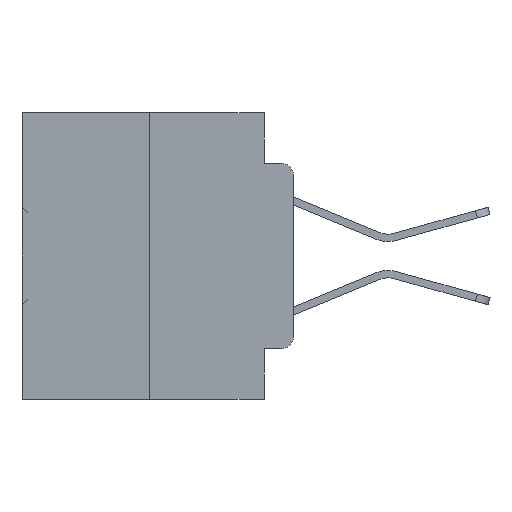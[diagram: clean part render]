
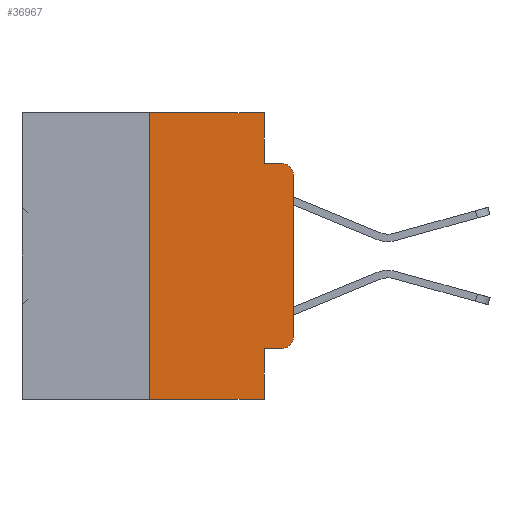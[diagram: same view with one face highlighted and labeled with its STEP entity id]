
A CAD part, left-side view. The second image highlights one B-rep face of the part: STEP entity #36967.
In plain terms, the highlighted planar face has unit normal (-1, 0, 0).
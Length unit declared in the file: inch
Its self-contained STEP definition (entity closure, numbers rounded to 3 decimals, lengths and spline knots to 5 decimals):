
#874 = AXIS2_PLACEMENT_3D ( 'NONE', #28032, #21718, #24745 ) ;
#1392 = VERTEX_POINT ( 'NONE', #15506 ) ;
#1552 = DIRECTION ( 'NONE',  ( 0., -1., 0. ) ) ;
#2329 = VERTEX_POINT ( 'NONE', #30217 ) ;
#2454 = CARTESIAN_POINT ( 'NONE',  ( 0., 0., 0. ) ) ;
#2911 = VECTOR ( 'NONE', #18882, 39.37008 ) ;
#3037 = ORIENTED_EDGE ( 'NONE', *, *, #19415, .F. ) ;
#3250 = CARTESIAN_POINT ( 'NONE',  ( 0., 0.473, -0.5 ) ) ;
#3820 = LINE ( 'NONE', #2454, #37466 ) ;
#4204 = PLANE ( 'NONE',  #874 ) ;
#4285 = CARTESIAN_POINT ( 'NONE',  ( 0., 0.051, -0.4115 ) ) ;
#6307 = ORIENTED_EDGE ( 'NONE', *, *, #28068, .T. ) ;
#7588 = LINE ( 'NONE', #27668, #2911 ) ;
#7749 = EDGE_CURVE ( 'NONE', #28274, #23318, #20915, .T. ) ;
#8713 = EDGE_CURVE ( 'NONE', #2329, #29225, #37156, .T. ) ;
#10219 = CARTESIAN_POINT ( 'NONE',  ( 0., 0., -0.1085 ) ) ;
#10695 = EDGE_CURVE ( 'NONE', #29225, #12432, #3820, .T. ) ;
#11150 = VECTOR ( 'NONE', #19279, 39.37008 ) ;
#11391 = CIRCLE ( 'NONE', #28610, 0.02 ) ;
#11540 = VECTOR ( 'NONE', #1552, 39.37008 ) ;
#11769 = CARTESIAN_POINT ( 'NONE',  ( 0., 0., -0.3915 ) ) ;
#12432 = VERTEX_POINT ( 'NONE', #10219 ) ;
#12592 = VERTEX_POINT ( 'NONE', #4285 ) ;
#12838 = CARTESIAN_POINT ( 'NONE',  ( 0., 0.051, -0.4115 ) ) ;
#12973 = LINE ( 'NONE', #37449, #19064 ) ;
#13054 = DIRECTION ( 'NONE',  ( 0., -1., 0. ) ) ;
#14446 = AXIS2_PLACEMENT_3D ( 'NONE', #26008, #37943, #20092 ) ;
#15447 = DIRECTION ( 'NONE',  ( 0., 0., -1. ) ) ;
#15506 = CARTESIAN_POINT ( 'NONE',  ( 0., 0.25, 0. ) ) ;
#15538 = ORIENTED_EDGE ( 'NONE', *, *, #36242, .F. ) ;
#16711 = DIRECTION ( 'NONE',  ( 0., -1., 0. ) ) ;
#17234 = LINE ( 'NONE', #12838, #11150 ) ;
#17476 = CARTESIAN_POINT ( 'NONE',  ( 0., 0.051, 0. ) ) ;
#18086 = ORIENTED_EDGE ( 'NONE', *, *, #10695, .T. ) ;
#18586 = VECTOR ( 'NONE', #32411, 39.37008 ) ;
#18787 = FACE_OUTER_BOUND ( 'NONE', #24685, .T. ) ;
#18882 = DIRECTION ( 'NONE',  ( 0., 0., 1. ) ) ;
#19064 = VECTOR ( 'NONE', #27180, 39.37008 ) ;
#19279 = DIRECTION ( 'NONE',  ( 0., -1., 0. ) ) ;
#19415 = EDGE_CURVE ( 'NONE', #12592, #24768, #23363, .T. ) ;
#20092 = DIRECTION ( 'NONE',  ( 0., 0., -1. ) ) ;
#20454 = VERTEX_POINT ( 'NONE', #21230 ) ;
#20861 = CARTESIAN_POINT ( 'NONE',  ( 0., 0.051, -0.0885 ) ) ;
#20915 = LINE ( 'NONE', #37309, #11540 ) ;
#21230 = CARTESIAN_POINT ( 'NONE',  ( 0., 0.051, 0. ) ) ;
#21705 = EDGE_CURVE ( 'NONE', #1392, #20454, #38519, .T. ) ;
#21718 = DIRECTION ( 'NONE',  ( 1., 0., 0. ) ) ;
#21783 = LINE ( 'NONE', #3250, #24646 ) ;
#21956 = ORIENTED_EDGE ( 'NONE', *, *, #24339, .T. ) ;
#22614 = CARTESIAN_POINT ( 'NONE',  ( 0., 0.25, -0.5 ) ) ;
#23318 = VERTEX_POINT ( 'NONE', #25498 ) ;
#23363 = LINE ( 'NONE', #17476, #18586 ) ;
#23574 = ORIENTED_EDGE ( 'NONE', *, *, #27005, .F. ) ;
#24339 = EDGE_CURVE ( 'NONE', #12432, #23318, #11391, .T. ) ;
#24366 = CARTESIAN_POINT ( 'NONE',  ( 0., 0.02, -0.1085 ) ) ;
#24646 = VECTOR ( 'NONE', #16711, 39.37008 ) ;
#24685 = EDGE_LOOP ( 'NONE', ( #18086, #21956, #36118, #23574, #37618, #15538, #6307, #3037, #32076, #35231 ) ) ;
#24745 = DIRECTION ( 'NONE',  ( 0., 0., -1. ) ) ;
#24768 = VERTEX_POINT ( 'NONE', #26286 ) ;
#25498 = CARTESIAN_POINT ( 'NONE',  ( 0., 0.02, -0.0885 ) ) ;
#26008 = CARTESIAN_POINT ( 'NONE',  ( 0., 0.02, -0.3915 ) ) ;
#26286 = CARTESIAN_POINT ( 'NONE',  ( 0., 0.051, -0.5 ) ) ;
#27005 = EDGE_CURVE ( 'NONE', #20454, #28274, #12973, .T. ) ;
#27180 = DIRECTION ( 'NONE',  ( 0., 0., -1. ) ) ;
#27269 = DIRECTION ( 'NONE',  ( -1., 0., 0. ) ) ;
#27668 = CARTESIAN_POINT ( 'NONE',  ( 0., 0.25, 0. ) ) ;
#28032 = CARTESIAN_POINT ( 'NONE',  ( 0., 0.473, 0. ) ) ;
#28068 = EDGE_CURVE ( 'NONE', #33722, #24768, #21783, .T. ) ;
#28274 = VERTEX_POINT ( 'NONE', #20861 ) ;
#28610 = AXIS2_PLACEMENT_3D ( 'NONE', #24366, #27269, #15447 ) ;
#28791 = VECTOR ( 'NONE', #13054, 39.37008 ) ;
#29225 = VERTEX_POINT ( 'NONE', #11769 ) ;
#30217 = CARTESIAN_POINT ( 'NONE',  ( 0., 0.02, -0.4115 ) ) ;
#32076 = ORIENTED_EDGE ( 'NONE', *, *, #32220, .T. ) ;
#32220 = EDGE_CURVE ( 'NONE', #12592, #2329, #17234, .T. ) ;
#32261 = DIRECTION ( 'NONE',  ( 0., 0., 1. ) ) ;
#32411 = DIRECTION ( 'NONE',  ( 0., 0., -1. ) ) ;
#33722 = VERTEX_POINT ( 'NONE', #22614 ) ;
#33739 = CARTESIAN_POINT ( 'NONE',  ( 0., 0.473, 0. ) ) ;
#35231 = ORIENTED_EDGE ( 'NONE', *, *, #8713, .T. ) ;
#36118 = ORIENTED_EDGE ( 'NONE', *, *, #7749, .F. ) ;
#36242 = EDGE_CURVE ( 'NONE', #33722, #1392, #7588, .T. ) ;
#36967 = ADVANCED_FACE ( 'NONE', ( #18787 ), #4204, .F. ) ;
#37156 = CIRCLE ( 'NONE', #14446, 0.02 ) ;
#37309 = CARTESIAN_POINT ( 'NONE',  ( 0., 0.051, -0.0885 ) ) ;
#37449 = CARTESIAN_POINT ( 'NONE',  ( 0., 0.051, 0. ) ) ;
#37466 = VECTOR ( 'NONE', #32261, 39.37008 ) ;
#37618 = ORIENTED_EDGE ( 'NONE', *, *, #21705, .F. ) ;
#37943 = DIRECTION ( 'NONE',  ( -1., 0., 0. ) ) ;
#38519 = LINE ( 'NONE', #33739, #28791 ) ;
